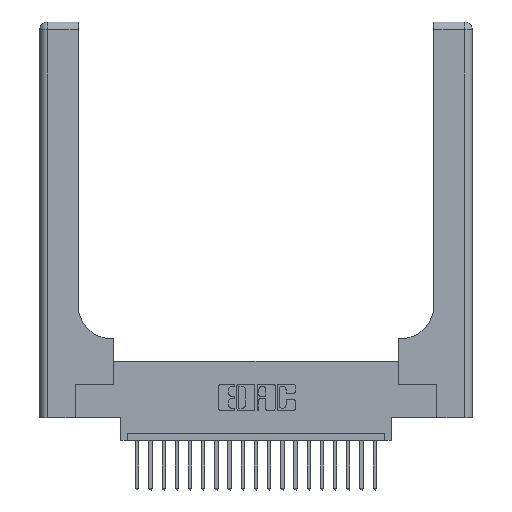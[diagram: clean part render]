
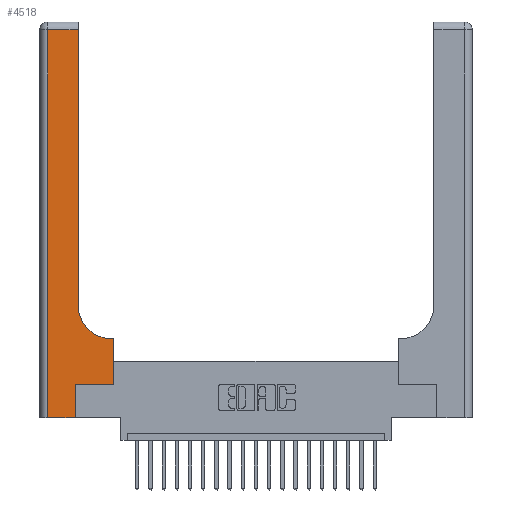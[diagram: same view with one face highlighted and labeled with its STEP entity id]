
A CAD part, top view. The second image highlights one B-rep face of the part: STEP entity #4518.
In plain terms, the highlighted planar face has unit normal (0, 0, 1).
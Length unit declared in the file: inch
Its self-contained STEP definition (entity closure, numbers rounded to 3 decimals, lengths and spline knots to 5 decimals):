
#1413 = EDGE_CURVE ( 'NONE', #9618, #6577, #14067, .T. ) ;
#2366 = CARTESIAN_POINT ( 'NONE',  ( 0.06, 3., 0.37 ) ) ;
#2399 = ORIENTED_EDGE ( 'NONE', *, *, #12709, .T. ) ;
#2440 = DIRECTION ( 'NONE',  ( 0., -1., 0. ) ) ;
#3210 = EDGE_LOOP ( 'NONE', ( #16862, #8873, #6582, #15494, #13208, #2399, #10973, #5282, #14524 ) ) ;
#3329 = CARTESIAN_POINT ( 'NONE',  ( 0.06, 0., 0.37 ) ) ;
#3575 = EDGE_CURVE ( 'NONE', #6354, #14190, #9879, .T. ) ;
#3966 = VECTOR ( 'NONE', #11036, 39.37008 ) ;
#4031 = DIRECTION ( 'NONE',  ( 0., 1., 0. ) ) ;
#4169 = VERTEX_POINT ( 'NONE', #15804 ) ;
#4289 = CARTESIAN_POINT ( 'NONE',  ( 0.2915, 0.6, 0.37 ) ) ;
#4340 = VECTOR ( 'NONE', #15072, 39.37008 ) ;
#4458 = PLANE ( 'NONE',  #22179 ) ;
#4518 = ADVANCED_FACE ( 'NONE', ( #14787 ), #4458, .F. ) ;
#5254 = CARTESIAN_POINT ( 'NONE',  ( 0.269, 0.25, 0.37 ) ) ;
#5282 = ORIENTED_EDGE ( 'NONE', *, *, #7790, .T. ) ;
#5919 = CARTESIAN_POINT ( 'NONE',  ( 0.2915, 3., 0.37 ) ) ;
#6354 = VERTEX_POINT ( 'NONE', #16732 ) ;
#6577 = VERTEX_POINT ( 'NONE', #6899 ) ;
#6582 = ORIENTED_EDGE ( 'NONE', *, *, #13632, .T. ) ;
#6890 = LINE ( 'NONE', #2366, #15700 ) ;
#6899 = CARTESIAN_POINT ( 'NONE',  ( 0.5585, 0.6, 0.37 ) ) ;
#7204 = CARTESIAN_POINT ( 'NONE',  ( 0.5585, 0.25, 0.37 ) ) ;
#7790 = EDGE_CURVE ( 'NONE', #6577, #6354, #11369, .T. ) ;
#7814 = CARTESIAN_POINT ( 'NONE',  ( 0.269, 0., 0.37 ) ) ;
#7921 = DIRECTION ( 'NONE',  ( 0., 0., -1. ) ) ;
#8435 = DIRECTION ( 'NONE',  ( 0., 0., -1. ) ) ;
#8717 = CARTESIAN_POINT ( 'NONE',  ( 0.269, 0., 0.37 ) ) ;
#8873 = ORIENTED_EDGE ( 'NONE', *, *, #21246, .T. ) ;
#9222 = VERTEX_POINT ( 'NONE', #3329 ) ;
#9618 = VERTEX_POINT ( 'NONE', #18387 ) ;
#9803 = DIRECTION ( 'NONE',  ( 0., 1., 0. ) ) ;
#9879 = CIRCLE ( 'NONE', #15527, 0.25 ) ;
#10193 = VERTEX_POINT ( 'NONE', #20303 ) ;
#10200 = LINE ( 'NONE', #5919, #18801 ) ;
#10230 = CARTESIAN_POINT ( 'NONE',  ( 0., 0., 0.37 ) ) ;
#10310 = DIRECTION ( 'NONE',  ( 1., 0., 0. ) ) ;
#10335 = LINE ( 'NONE', #7814, #4340 ) ;
#10973 = ORIENTED_EDGE ( 'NONE', *, *, #1413, .T. ) ;
#11036 = DIRECTION ( 'NONE',  ( -1., 0., 0. ) ) ;
#11369 = LINE ( 'NONE', #4289, #3966 ) ;
#11571 = EDGE_CURVE ( 'NONE', #14173, #4169, #10335, .T. ) ;
#11952 = CARTESIAN_POINT ( 'NONE',  ( 0.5415, 0.85, 0.37 ) ) ;
#12170 = VECTOR ( 'NONE', #4031, 39.37008 ) ;
#12709 = EDGE_CURVE ( 'NONE', #4169, #9618, #12993, .T. ) ;
#12788 = LINE ( 'NONE', #10230, #14427 ) ;
#12993 = LINE ( 'NONE', #5254, #20744 ) ;
#13010 = EDGE_CURVE ( 'NONE', #14190, #10193, #10200, .T. ) ;
#13208 = ORIENTED_EDGE ( 'NONE', *, *, #11571, .T. ) ;
#13632 = EDGE_CURVE ( 'NONE', #22159, #9222, #6890, .T. ) ;
#13768 = CARTESIAN_POINT ( 'NONE',  ( 0.06, 2.94, 0.37 ) ) ;
#13771 = DIRECTION ( 'NONE',  ( 1., 0., 0. ) ) ;
#14067 = LINE ( 'NONE', #7204, #12170 ) ;
#14173 = VERTEX_POINT ( 'NONE', #8717 ) ;
#14190 = VERTEX_POINT ( 'NONE', #22755 ) ;
#14427 = VECTOR ( 'NONE', #10310, 39.37008 ) ;
#14524 = ORIENTED_EDGE ( 'NONE', *, *, #3575, .T. ) ;
#14787 = FACE_OUTER_BOUND ( 'NONE', #3210, .T. ) ;
#14816 = CARTESIAN_POINT ( 'NONE',  ( 0., 2.94, 0.37 ) ) ;
#15048 = DIRECTION ( 'NONE',  ( -1., 0., 0. ) ) ;
#15072 = DIRECTION ( 'NONE',  ( 0., 1., 0. ) ) ;
#15494 = ORIENTED_EDGE ( 'NONE', *, *, #18006, .T. ) ;
#15527 = AXIS2_PLACEMENT_3D ( 'NONE', #11952, #8435, #13771 ) ;
#15700 = VECTOR ( 'NONE', #2440, 39.37008 ) ;
#15804 = CARTESIAN_POINT ( 'NONE',  ( 0.269, 0.25, 0.37 ) ) ;
#16445 = DIRECTION ( 'NONE',  ( -1., 0., 0. ) ) ;
#16732 = CARTESIAN_POINT ( 'NONE',  ( 0.5415, 0.6, 0.37 ) ) ;
#16862 = ORIENTED_EDGE ( 'NONE', *, *, #13010, .T. ) ;
#17365 = LINE ( 'NONE', #14816, #21495 ) ;
#17562 = DIRECTION ( 'NONE',  ( 1., 0., 0. ) ) ;
#18006 = EDGE_CURVE ( 'NONE', #9222, #14173, #12788, .T. ) ;
#18387 = CARTESIAN_POINT ( 'NONE',  ( 0.5585, 0.25, 0.37 ) ) ;
#18521 = CARTESIAN_POINT ( 'NONE',  ( 0., 3., 0.37 ) ) ;
#18801 = VECTOR ( 'NONE', #9803, 39.37008 ) ;
#20303 = CARTESIAN_POINT ( 'NONE',  ( 0.2915, 2.94, 0.37 ) ) ;
#20744 = VECTOR ( 'NONE', #17562, 39.37008 ) ;
#21246 = EDGE_CURVE ( 'NONE', #10193, #22159, #17365, .T. ) ;
#21495 = VECTOR ( 'NONE', #15048, 39.37008 ) ;
#22159 = VERTEX_POINT ( 'NONE', #13768 ) ;
#22179 = AXIS2_PLACEMENT_3D ( 'NONE', #18521, #7921, #16445 ) ;
#22755 = CARTESIAN_POINT ( 'NONE',  ( 0.2915, 0.85, 0.37 ) ) ;
